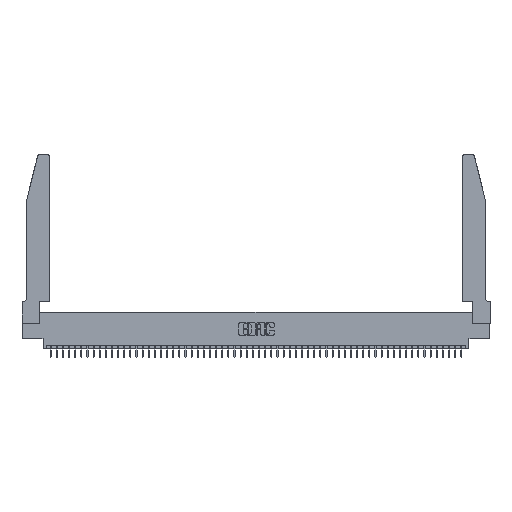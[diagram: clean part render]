
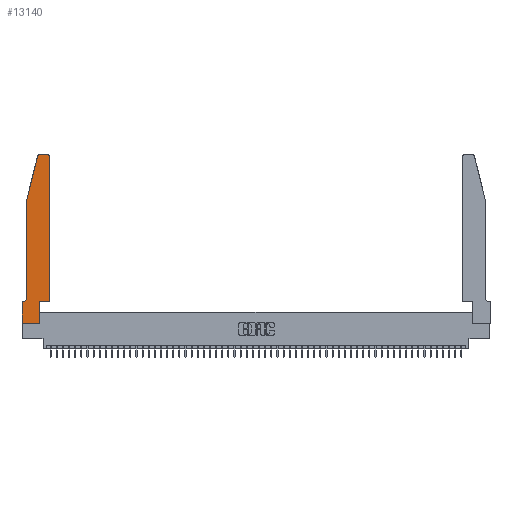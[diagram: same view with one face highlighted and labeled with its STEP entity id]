
A CAD part, top view. The second image highlights one B-rep face of the part: STEP entity #13140.
In plain terms, the highlighted planar face has unit normal (0, 0, 1).
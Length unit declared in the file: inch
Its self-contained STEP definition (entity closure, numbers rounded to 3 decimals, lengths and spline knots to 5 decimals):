
#121 = VECTOR ( 'NONE', #29432, 39.37008 ) ;
#230 = EDGE_CURVE ( 'NONE', #15300, #15210, #36473, .T. ) ;
#272 = VERTEX_POINT ( 'NONE', #48100 ) ;
#2547 = ORIENTED_EDGE ( 'NONE', *, *, #26080, .T. ) ;
#3811 = CIRCLE ( 'NONE', #43759, 0.03 ) ;
#4070 = ORIENTED_EDGE ( 'NONE', *, *, #48705, .T. ) ;
#4165 = CARTESIAN_POINT ( 'NONE',  ( 0.0755, 0.35, 0.37 ) ) ;
#4367 = LINE ( 'NONE', #28818, #33115 ) ;
#4439 = LINE ( 'NONE', #4165, #121 ) ;
#4813 = CARTESIAN_POINT ( 'NONE',  ( 0., 0., 0.37 ) ) ;
#4903 = DIRECTION ( 'NONE',  ( 0., 0., -1. ) ) ;
#5498 = CARTESIAN_POINT ( 'NONE',  ( 0.0755, 2., 0.37 ) ) ;
#7185 = LINE ( 'NONE', #11077, #39390 ) ;
#7259 = VECTOR ( 'NONE', #26677, 39.37008 ) ;
#7298 = AXIS2_PLACEMENT_3D ( 'NONE', #19143, #22762, #27474 ) ;
#7377 = VECTOR ( 'NONE', #11710, 39.37008 ) ;
#7553 = CARTESIAN_POINT ( 'NONE',  ( 0., 0.35, 0.37 ) ) ;
#8094 = DIRECTION ( 'NONE',  ( 1., 0., 0. ) ) ;
#8205 = VECTOR ( 'NONE', #48130, 39.37008 ) ;
#8482 = CARTESIAN_POINT ( 'NONE',  ( 0.4505, 0.35, 0.37 ) ) ;
#8949 = EDGE_CURVE ( 'NONE', #27967, #15300, #42875, .T. ) ;
#9663 = LINE ( 'NONE', #5498, #25308 ) ;
#10891 = CARTESIAN_POINT ( 'NONE',  ( 0., 0., 0.37 ) ) ;
#11077 = CARTESIAN_POINT ( 'NONE',  ( 0.0755, 2., 0.37 ) ) ;
#11710 = DIRECTION ( 'NONE',  ( 0., -1., 0. ) ) ;
#11852 = ORIENTED_EDGE ( 'NONE', *, *, #33501, .T. ) ;
#12046 = ORIENTED_EDGE ( 'NONE', *, *, #230, .T. ) ;
#12267 = PLANE ( 'NONE',  #39180 ) ;
#12461 = VERTEX_POINT ( 'NONE', #54339 ) ;
#13140 = ADVANCED_FACE ( 'NONE', ( #33374 ), #12267, .T. ) ;
#14120 = CIRCLE ( 'NONE', #48725, 0.07 ) ;
#14242 = CARTESIAN_POINT ( 'NONE',  ( 0.0055, 0.35, 0.37 ) ) ;
#15084 = CARTESIAN_POINT ( 'NONE',  ( 0.0755, 0.42, 0.37 ) ) ;
#15210 = VERTEX_POINT ( 'NONE', #33785 ) ;
#15300 = VERTEX_POINT ( 'NONE', #52413 ) ;
#16740 = VERTEX_POINT ( 'NONE', #15084 ) ;
#16952 = EDGE_LOOP ( 'NONE', ( #33991, #22590, #27114, #52299, #24968, #45011, #2547, #34586, #12046, #46762, #4070, #11852 ) ) ;
#17141 = DIRECTION ( 'NONE',  ( 0., 1., 0. ) ) ;
#17597 = DIRECTION ( 'NONE',  ( 1., 0., 0. ) ) ;
#17693 = VECTOR ( 'NONE', #17597, 39.37008 ) ;
#18298 = VERTEX_POINT ( 'NONE', #14242 ) ;
#18634 = LINE ( 'NONE', #40009, #7259 ) ;
#19143 = CARTESIAN_POINT ( 'NONE',  ( 0.4205, 2.72, 0.37 ) ) ;
#19202 = EDGE_CURVE ( 'NONE', #272, #16740, #9663, .T. ) ;
#19727 = CIRCLE ( 'NONE', #7298, 0.03 ) ;
#22457 = DIRECTION ( 'NONE',  ( 0., -1., 0. ) ) ;
#22590 = ORIENTED_EDGE ( 'NONE', *, *, #48701, .T. ) ;
#22607 = VERTEX_POINT ( 'NONE', #24170 ) ;
#22762 = DIRECTION ( 'NONE',  ( 0., 0., 1. ) ) ;
#23080 = VERTEX_POINT ( 'NONE', #28517 ) ;
#24170 = CARTESIAN_POINT ( 'NONE',  ( 0.4205, 2.75, 0.37 ) ) ;
#24506 = DIRECTION ( 'NONE',  ( 0., 0., 1. ) ) ;
#24968 = ORIENTED_EDGE ( 'NONE', *, *, #43313, .T. ) ;
#25308 = VECTOR ( 'NONE', #22457, 39.37008 ) ;
#26080 = EDGE_CURVE ( 'NONE', #43487, #27967, #36454, .T. ) ;
#26350 = CARTESIAN_POINT ( 'NONE',  ( 0., 0., 0.37 ) ) ;
#26677 = DIRECTION ( 'NONE',  ( 1., 0., 0. ) ) ;
#27114 = ORIENTED_EDGE ( 'NONE', *, *, #49840, .T. ) ;
#27474 = DIRECTION ( 'NONE',  ( 1., 0., 0. ) ) ;
#27967 = VERTEX_POINT ( 'NONE', #26350 ) ;
#28517 = CARTESIAN_POINT ( 'NONE',  ( 0.25487, 2.72718, 0.37 ) ) ;
#28818 = CARTESIAN_POINT ( 'NONE',  ( 0.4505, 0.35, 0.37 ) ) ;
#29432 = DIRECTION ( 'NONE',  ( -1., 0., 0. ) ) ;
#30052 = EDGE_CURVE ( 'NONE', #18298, #43487, #4439, .T. ) ;
#30453 = DIRECTION ( 'NONE',  ( -1., 0., 0. ) ) ;
#31150 = CARTESIAN_POINT ( 'NONE',  ( 0.2605, 2.75, 0.37 ) ) ;
#32199 = DIRECTION ( 'NONE',  ( -0.239, -0.971, 0. ) ) ;
#32312 = DIRECTION ( 'NONE',  ( 0., 1., 0. ) ) ;
#32656 = EDGE_CURVE ( 'NONE', #15210, #36875, #18634, .T. ) ;
#33115 = VECTOR ( 'NONE', #17141, 39.37008 ) ;
#33270 = DIRECTION ( 'NONE',  ( 0., 0., 1. ) ) ;
#33374 = FACE_OUTER_BOUND ( 'NONE', #16952, .T. ) ;
#33501 = EDGE_CURVE ( 'NONE', #12461, #22607, #19727, .T. ) ;
#33785 = CARTESIAN_POINT ( 'NONE',  ( 0.2865, 0.35, 0.37 ) ) ;
#33792 = CARTESIAN_POINT ( 'NONE',  ( 0.0055, 0.42, 0.37 ) ) ;
#33991 = ORIENTED_EDGE ( 'NONE', *, *, #48049, .T. ) ;
#34586 = ORIENTED_EDGE ( 'NONE', *, *, #8949, .T. ) ;
#35082 = VECTOR ( 'NONE', #32312, 39.37008 ) ;
#36454 = LINE ( 'NONE', #10891, #7377 ) ;
#36473 = LINE ( 'NONE', #53436, #35082 ) ;
#36875 = VERTEX_POINT ( 'NONE', #8482 ) ;
#39180 = AXIS2_PLACEMENT_3D ( 'NONE', #7553, #24506, #8094 ) ;
#39390 = VECTOR ( 'NONE', #32199, 39.37008 ) ;
#40009 = CARTESIAN_POINT ( 'NONE',  ( 0.4505, 0.35, 0.37 ) ) ;
#40187 = CARTESIAN_POINT ( 'NONE',  ( 0., 0.35, 0.37 ) ) ;
#42427 = DIRECTION ( 'NONE',  ( 1., 0., 0. ) ) ;
#42875 = LINE ( 'NONE', #4813, #17693 ) ;
#43313 = EDGE_CURVE ( 'NONE', #16740, #18298, #14120, .T. ) ;
#43487 = VERTEX_POINT ( 'NONE', #40187 ) ;
#43759 = AXIS2_PLACEMENT_3D ( 'NONE', #46064, #33270, #42427 ) ;
#44229 = LINE ( 'NONE', #31150, #8205 ) ;
#45011 = ORIENTED_EDGE ( 'NONE', *, *, #30052, .T. ) ;
#46064 = CARTESIAN_POINT ( 'NONE',  ( 0.284, 2.72, 0.37 ) ) ;
#46762 = ORIENTED_EDGE ( 'NONE', *, *, #32656, .T. ) ;
#47604 = VERTEX_POINT ( 'NONE', #49821 ) ;
#48049 = EDGE_CURVE ( 'NONE', #22607, #47604, #44229, .T. ) ;
#48100 = CARTESIAN_POINT ( 'NONE',  ( 0.0755, 2., 0.37 ) ) ;
#48130 = DIRECTION ( 'NONE',  ( -1., 0., 0. ) ) ;
#48701 = EDGE_CURVE ( 'NONE', #47604, #23080, #3811, .T. ) ;
#48705 = EDGE_CURVE ( 'NONE', #36875, #12461, #4367, .T. ) ;
#48725 = AXIS2_PLACEMENT_3D ( 'NONE', #33792, #4903, #30453 ) ;
#49821 = CARTESIAN_POINT ( 'NONE',  ( 0.284, 2.75, 0.37 ) ) ;
#49840 = EDGE_CURVE ( 'NONE', #23080, #272, #7185, .T. ) ;
#52299 = ORIENTED_EDGE ( 'NONE', *, *, #19202, .T. ) ;
#52413 = CARTESIAN_POINT ( 'NONE',  ( 0.2865, 0., 0.37 ) ) ;
#53436 = CARTESIAN_POINT ( 'NONE',  ( 0.2865, 0.35, 0.37 ) ) ;
#54339 = CARTESIAN_POINT ( 'NONE',  ( 0.4505, 2.72, 0.37 ) ) ;
